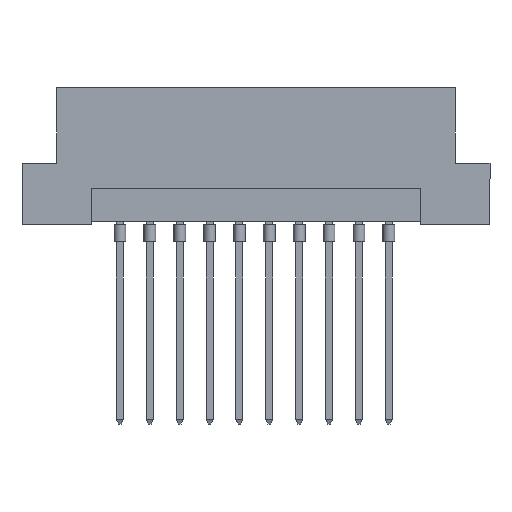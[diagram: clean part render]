
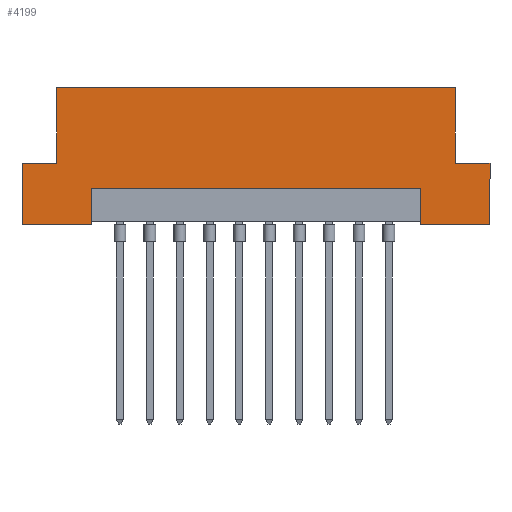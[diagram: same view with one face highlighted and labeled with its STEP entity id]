
A CAD part, front view. The second image highlights one B-rep face of the part: STEP entity #4199.
In plain terms, the highlighted planar face has unit normal (0, -1, 0).
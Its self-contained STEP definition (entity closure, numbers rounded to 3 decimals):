
#41 = VECTOR ( 'NONE', #5063, 1000. ) ;
#94 = CARTESIAN_POINT ( 'NONE',  ( -14., -4.3, 3. ) ) ;
#163 = EDGE_CURVE ( 'NONE', #911, #4396, #883, .T. ) ;
#179 = CARTESIAN_POINT ( 'NONE',  ( 19.9, -4.3, 0. ) ) ;
#240 = EDGE_CURVE ( 'NONE', #273, #4396, #5310, .T. ) ;
#273 = VERTEX_POINT ( 'NONE', #5340 ) ;
#305 = VECTOR ( 'NONE', #4414, 1000. ) ;
#379 = LINE ( 'NONE', #5579, #4098 ) ;
#448 = CARTESIAN_POINT ( 'NONE',  ( -16.94, -4.3, 11.6 ) ) ;
#487 = EDGE_CURVE ( 'NONE', #2357, #4417, #3339, .T. ) ;
#559 = LINE ( 'NONE', #2341, #702 ) ;
#599 = CARTESIAN_POINT ( 'NONE',  ( 14., -4.3, 0.2 ) ) ;
#679 = CARTESIAN_POINT ( 'NONE',  ( -19.9, -4.3, 11.6 ) ) ;
#702 = VECTOR ( 'NONE', #1007, 1000. ) ;
#850 = EDGE_CURVE ( 'NONE', #2357, #4766, #1080, .T. ) ;
#883 = LINE ( 'NONE', #2187, #1434 ) ;
#885 = ORIENTED_EDGE ( 'NONE', *, *, #3466, .T. ) ;
#902 = EDGE_CURVE ( 'NONE', #4547, #1257, #4383, .T. ) ;
#911 = VERTEX_POINT ( 'NONE', #94 ) ;
#1007 = DIRECTION ( 'NONE',  ( 0., 0., 1. ) ) ;
#1080 = LINE ( 'NONE', #599, #1783 ) ;
#1250 = ORIENTED_EDGE ( 'NONE', *, *, #487, .T. ) ;
#1257 = VERTEX_POINT ( 'NONE', #448 ) ;
#1332 = EDGE_CURVE ( 'NONE', #3387, #273, #4648, .T. ) ;
#1377 = DIRECTION ( 'NONE',  ( 1., 0., 0. ) ) ;
#1420 = LINE ( 'NONE', #4068, #2233 ) ;
#1434 = VECTOR ( 'NONE', #3584, 1000. ) ;
#1512 = LINE ( 'NONE', #5019, #4373 ) ;
#1545 = DIRECTION ( 'NONE',  ( 0., 0., -1. ) ) ;
#1604 = VECTOR ( 'NONE', #1545, 1000. ) ;
#1648 = EDGE_CURVE ( 'NONE', #3236, #4417, #379, .T. ) ;
#1671 = CARTESIAN_POINT ( 'NONE',  ( 14., -4.3, 3. ) ) ;
#1679 = CARTESIAN_POINT ( 'NONE',  ( 14., -4.3, 0. ) ) ;
#1783 = VECTOR ( 'NONE', #3283, 1000. ) ;
#1934 = CARTESIAN_POINT ( 'NONE',  ( 19.9, -4.3, 11.6 ) ) ;
#2146 = AXIS2_PLACEMENT_3D ( 'NONE', #1934, #4665, #2448 ) ;
#2167 = EDGE_LOOP ( 'NONE', ( #3511, #2986, #1250, #3733, #2784, #885, #3272, #3829, #5170, #5496, #3237, #4281 ) ) ;
#2177 = CARTESIAN_POINT ( 'NONE',  ( 19.9, -4.3, 5.2 ) ) ;
#2187 = CARTESIAN_POINT ( 'NONE',  ( -14., -4.3, 0.2 ) ) ;
#2233 = VECTOR ( 'NONE', #5390, 1000. ) ;
#2269 = CARTESIAN_POINT ( 'NONE',  ( 19.9, -4.3, 0. ) ) ;
#2341 = CARTESIAN_POINT ( 'NONE',  ( 16.94, -4.3, 5.2 ) ) ;
#2343 = EDGE_CURVE ( 'NONE', #5497, #3236, #5187, .T. ) ;
#2357 = VERTEX_POINT ( 'NONE', #1679 ) ;
#2448 = DIRECTION ( 'NONE',  ( -1., 0., 0. ) ) ;
#2520 = EDGE_CURVE ( 'NONE', #3387, #4547, #1420, .T. ) ;
#2533 = CARTESIAN_POINT ( 'NONE',  ( -14., -4.3, 0. ) ) ;
#2690 = VECTOR ( 'NONE', #3547, 1000. ) ;
#2784 = ORIENTED_EDGE ( 'NONE', *, *, #2343, .F. ) ;
#2986 = ORIENTED_EDGE ( 'NONE', *, *, #850, .F. ) ;
#3065 = CARTESIAN_POINT ( 'NONE',  ( -16.94, -4.3, 5.2 ) ) ;
#3236 = VERTEX_POINT ( 'NONE', #3467 ) ;
#3237 = ORIENTED_EDGE ( 'NONE', *, *, #240, .T. ) ;
#3272 = ORIENTED_EDGE ( 'NONE', *, *, #4001, .F. ) ;
#3283 = DIRECTION ( 'NONE',  ( 0., 0., 1. ) ) ;
#3337 = FACE_OUTER_BOUND ( 'NONE', #2167, .T. ) ;
#3339 = LINE ( 'NONE', #179, #41 ) ;
#3387 = VERTEX_POINT ( 'NONE', #4330 ) ;
#3466 = EDGE_CURVE ( 'NONE', #5497, #4991, #559, .T. ) ;
#3467 = CARTESIAN_POINT ( 'NONE',  ( 19.9, -4.3, 5.2 ) ) ;
#3511 = ORIENTED_EDGE ( 'NONE', *, *, #3583, .T. ) ;
#3547 = DIRECTION ( 'NONE',  ( 1., 0., 0. ) ) ;
#3583 = EDGE_CURVE ( 'NONE', #911, #4766, #1512, .T. ) ;
#3584 = DIRECTION ( 'NONE',  ( 0., 0., -1. ) ) ;
#3733 = ORIENTED_EDGE ( 'NONE', *, *, #1648, .F. ) ;
#3829 = ORIENTED_EDGE ( 'NONE', *, *, #902, .F. ) ;
#4001 = EDGE_CURVE ( 'NONE', #1257, #4991, #4520, .T. ) ;
#4068 = CARTESIAN_POINT ( 'NONE',  ( -19.9, -4.3, 5.2 ) ) ;
#4098 = VECTOR ( 'NONE', #4349, 1000. ) ;
#4199 = ADVANCED_FACE ( 'NONE', ( #3337 ), #4635, .F. ) ;
#4281 = ORIENTED_EDGE ( 'NONE', *, *, #163, .F. ) ;
#4330 = CARTESIAN_POINT ( 'NONE',  ( -19.9, -4.3, 5.2 ) ) ;
#4349 = DIRECTION ( 'NONE',  ( 0., 0., -1. ) ) ;
#4373 = VECTOR ( 'NONE', #4443, 1000. ) ;
#4383 = LINE ( 'NONE', #3065, #305 ) ;
#4396 = VERTEX_POINT ( 'NONE', #2533 ) ;
#4414 = DIRECTION ( 'NONE',  ( 0., 0., 1. ) ) ;
#4417 = VERTEX_POINT ( 'NONE', #4431 ) ;
#4431 = CARTESIAN_POINT ( 'NONE',  ( 19.9, -4.3, 0. ) ) ;
#4439 = VECTOR ( 'NONE', #5262, 1000. ) ;
#4443 = DIRECTION ( 'NONE',  ( 1., 0., 0. ) ) ;
#4480 = CARTESIAN_POINT ( 'NONE',  ( 16.94, -4.3, 11.6 ) ) ;
#4495 = CARTESIAN_POINT ( 'NONE',  ( 16.94, -4.3, 5.2 ) ) ;
#4520 = LINE ( 'NONE', #4891, #2690 ) ;
#4547 = VERTEX_POINT ( 'NONE', #4640 ) ;
#4635 = PLANE ( 'NONE',  #2146 ) ;
#4640 = CARTESIAN_POINT ( 'NONE',  ( -16.94, -4.3, 5.2 ) ) ;
#4648 = LINE ( 'NONE', #679, #1604 ) ;
#4665 = DIRECTION ( 'NONE',  ( 0., 1., 0. ) ) ;
#4766 = VERTEX_POINT ( 'NONE', #1671 ) ;
#4891 = CARTESIAN_POINT ( 'NONE',  ( 19.9, -4.3, 11.6 ) ) ;
#4991 = VERTEX_POINT ( 'NONE', #4480 ) ;
#5019 = CARTESIAN_POINT ( 'NONE',  ( -14., -4.3, 3. ) ) ;
#5063 = DIRECTION ( 'NONE',  ( 1., 0., 0. ) ) ;
#5170 = ORIENTED_EDGE ( 'NONE', *, *, #2520, .F. ) ;
#5187 = LINE ( 'NONE', #2177, #4439 ) ;
#5262 = DIRECTION ( 'NONE',  ( 1., 0., 0. ) ) ;
#5286 = VECTOR ( 'NONE', #1377, 1000. ) ;
#5310 = LINE ( 'NONE', #2269, #5286 ) ;
#5340 = CARTESIAN_POINT ( 'NONE',  ( -19.9, -4.3, 0. ) ) ;
#5390 = DIRECTION ( 'NONE',  ( 1., 0., 0. ) ) ;
#5496 = ORIENTED_EDGE ( 'NONE', *, *, #1332, .T. ) ;
#5497 = VERTEX_POINT ( 'NONE', #4495 ) ;
#5579 = CARTESIAN_POINT ( 'NONE',  ( 19.9, -4.3, 11.6 ) ) ;
